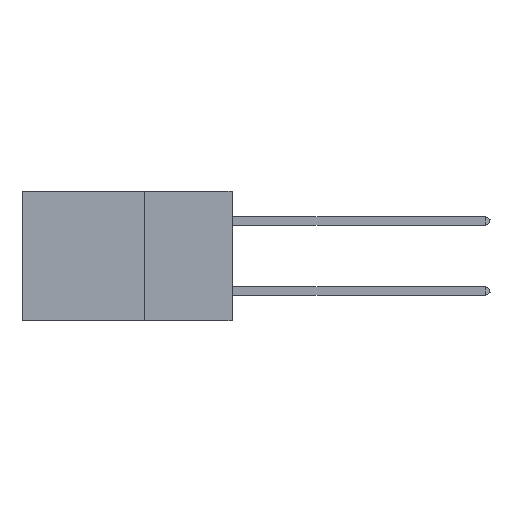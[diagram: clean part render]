
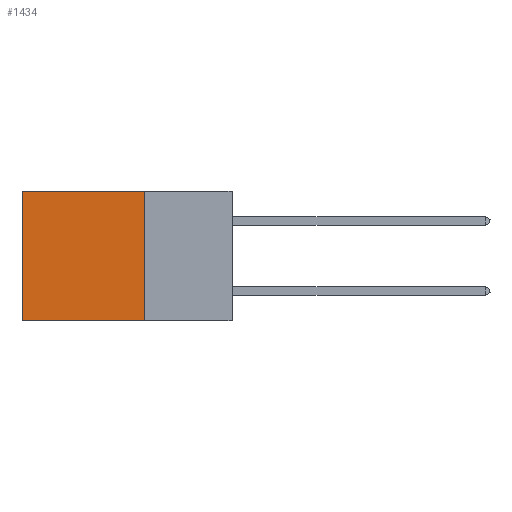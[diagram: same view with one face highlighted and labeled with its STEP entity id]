
A CAD part, left-side view. The second image highlights one B-rep face of the part: STEP entity #1434.
In plain terms, the highlighted planar face has unit normal (-1, 0, 0).
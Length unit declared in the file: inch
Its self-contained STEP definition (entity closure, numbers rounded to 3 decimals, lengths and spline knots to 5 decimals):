
#752 = CARTESIAN_POINT ( 'NONE',  ( 0.2875, 0.6, 0. ) ) ;
#1434 = ADVANCED_FACE ( 'NONE', ( #13910 ), #13739, .F. ) ;
#1685 = VECTOR ( 'NONE', #24257, 39.37008 ) ;
#3762 = EDGE_LOOP ( 'NONE', ( #32278, #30213, #5829, #6588 ) ) ;
#5829 = ORIENTED_EDGE ( 'NONE', *, *, #32285, .F. ) ;
#6588 = ORIENTED_EDGE ( 'NONE', *, *, #13834, .T. ) ;
#6988 = AXIS2_PLACEMENT_3D ( 'NONE', #11512, #19565, #13978 ) ;
#8167 = VERTEX_POINT ( 'NONE', #8583 ) ;
#8583 = CARTESIAN_POINT ( 'NONE',  ( 0.2875, 0.25, 0. ) ) ;
#9725 = LINE ( 'NONE', #25961, #30485 ) ;
#11512 = CARTESIAN_POINT ( 'NONE',  ( 0.2875, 0.25, 0. ) ) ;
#13739 = PLANE ( 'NONE',  #6988 ) ;
#13834 = EDGE_CURVE ( 'NONE', #8167, #31352, #21954, .T. ) ;
#13910 = FACE_OUTER_BOUND ( 'NONE', #3762, .T. ) ;
#13978 = DIRECTION ( 'NONE',  ( 0., 0., -1. ) ) ;
#14938 = CARTESIAN_POINT ( 'NONE',  ( 0.2875, 0.25, 0. ) ) ;
#15157 = CARTESIAN_POINT ( 'NONE',  ( 0.2875, 0.25, -0.37 ) ) ;
#15513 = VECTOR ( 'NONE', #32158, 39.37008 ) ;
#16069 = CARTESIAN_POINT ( 'NONE',  ( 0.2875, 0.6, 0. ) ) ;
#16448 = LINE ( 'NONE', #16069, #1685 ) ;
#18142 = DIRECTION ( 'NONE',  ( 0., 1., 0. ) ) ;
#19565 = DIRECTION ( 'NONE',  ( 1., 0., 0. ) ) ;
#19949 = DIRECTION ( 'NONE',  ( 0., 0., -1. ) ) ;
#21336 = CARTESIAN_POINT ( 'NONE',  ( 0.2875, 0.25, 0. ) ) ;
#21954 = LINE ( 'NONE', #21336, #15513 ) ;
#23217 = CARTESIAN_POINT ( 'NONE',  ( 0.2875, 0.6, -0.37 ) ) ;
#24257 = DIRECTION ( 'NONE',  ( 0., 0., -1. ) ) ;
#25961 = CARTESIAN_POINT ( 'NONE',  ( 0.2875, 0.25, -0.37 ) ) ;
#27467 = VECTOR ( 'NONE', #19949, 39.37008 ) ;
#28044 = VERTEX_POINT ( 'NONE', #15157 ) ;
#29722 = VERTEX_POINT ( 'NONE', #23217 ) ;
#30213 = ORIENTED_EDGE ( 'NONE', *, *, #32315, .F. ) ;
#30485 = VECTOR ( 'NONE', #18142, 39.37008 ) ;
#31352 = VERTEX_POINT ( 'NONE', #752 ) ;
#32158 = DIRECTION ( 'NONE',  ( 0., 1., 0. ) ) ;
#32278 = ORIENTED_EDGE ( 'NONE', *, *, #32774, .T. ) ;
#32285 = EDGE_CURVE ( 'NONE', #8167, #28044, #34638, .T. ) ;
#32315 = EDGE_CURVE ( 'NONE', #28044, #29722, #9725, .T. ) ;
#32774 = EDGE_CURVE ( 'NONE', #31352, #29722, #16448, .T. ) ;
#34638 = LINE ( 'NONE', #14938, #27467 ) ;
